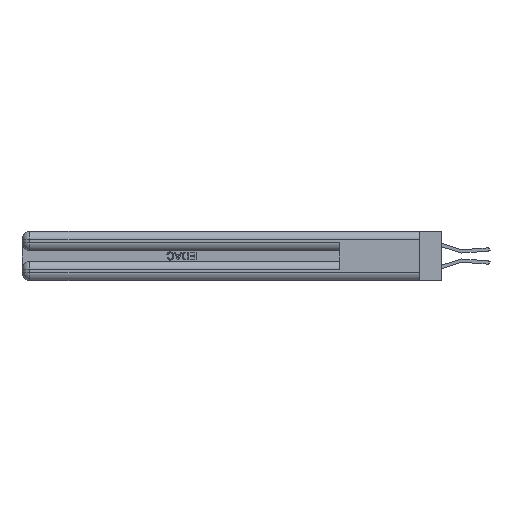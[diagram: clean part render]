
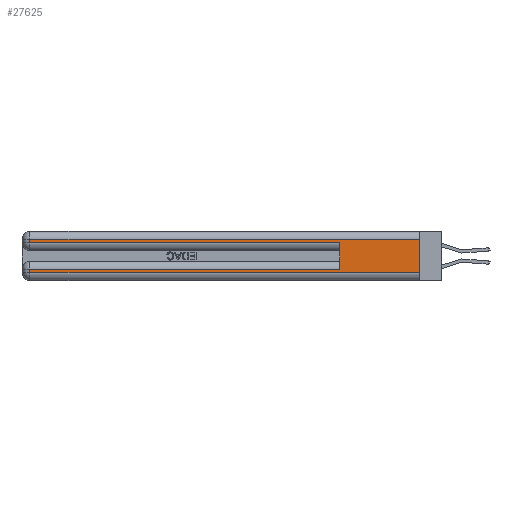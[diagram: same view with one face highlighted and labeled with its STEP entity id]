
A CAD part, left-side view. The second image highlights one B-rep face of the part: STEP entity #27625.
In plain terms, the highlighted planar face has unit normal (-1, 0, 0).
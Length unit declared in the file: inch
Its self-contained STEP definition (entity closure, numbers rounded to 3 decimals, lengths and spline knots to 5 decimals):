
#593 = VECTOR ( 'NONE', #5340, 39.37008 ) ;
#1022 = EDGE_CURVE ( 'NONE', #13051, #31233, #8066, .T. ) ;
#1693 = LINE ( 'NONE', #26097, #593 ) ;
#4827 = LINE ( 'NONE', #14614, #22151 ) ;
#4850 = CARTESIAN_POINT ( 'NONE',  ( 0., 0., 0.06 ) ) ;
#5340 = DIRECTION ( 'NONE',  ( 0., 0., -1. ) ) ;
#6098 = VECTOR ( 'NONE', #33694, 39.37008 ) ;
#6154 = ORIENTED_EDGE ( 'NONE', *, *, #6238, .T. ) ;
#6183 = VECTOR ( 'NONE', #44183, 39.37008 ) ;
#6238 = EDGE_CURVE ( 'NONE', #12537, #31115, #41715, .T. ) ;
#7185 = EDGE_CURVE ( 'NONE', #34861, #31233, #4827, .T. ) ;
#8066 = LINE ( 'NONE', #21139, #43744 ) ;
#8186 = ORIENTED_EDGE ( 'NONE', *, *, #37562, .F. ) ;
#10264 = CARTESIAN_POINT ( 'NONE',  ( 0., 0., 0.37 ) ) ;
#10406 = EDGE_LOOP ( 'NONE', ( #8186, #20085, #37996, #13645, #25565, #37518, #39146, #6154 ) ) ;
#10673 = VERTEX_POINT ( 'NONE', #22698 ) ;
#10731 = VERTEX_POINT ( 'NONE', #16223 ) ;
#11060 = CARTESIAN_POINT ( 'NONE',  ( 0., 2.94, 0.37 ) ) ;
#12537 = VERTEX_POINT ( 'NONE', #40251 ) ;
#13051 = VERTEX_POINT ( 'NONE', #29453 ) ;
#13645 = ORIENTED_EDGE ( 'NONE', *, *, #7185, .T. ) ;
#14118 = CARTESIAN_POINT ( 'NONE',  ( 0., 0., 0.085 ) ) ;
#14153 = VECTOR ( 'NONE', #23582, 39.37008 ) ;
#14243 = LINE ( 'NONE', #26737, #6098 ) ;
#14614 = CARTESIAN_POINT ( 'NONE',  ( 0., 0., 0.285 ) ) ;
#16223 = CARTESIAN_POINT ( 'NONE',  ( 0., 0., 0.31 ) ) ;
#16676 = CARTESIAN_POINT ( 'NONE',  ( 0., 2.94, 0.31 ) ) ;
#16988 = EDGE_CURVE ( 'NONE', #10673, #12537, #40811, .T. ) ;
#20000 = CARTESIAN_POINT ( 'NONE',  ( 0., 2.94, 0.37 ) ) ;
#20085 = ORIENTED_EDGE ( 'NONE', *, *, #32410, .T. ) ;
#20654 = DIRECTION ( 'NONE',  ( 1., 0., 0. ) ) ;
#21139 = CARTESIAN_POINT ( 'NONE',  ( 0., 0.6, 0.145 ) ) ;
#22151 = VECTOR ( 'NONE', #28343, 39.37008 ) ;
#22698 = CARTESIAN_POINT ( 'NONE',  ( 0., 2.94, 0.085 ) ) ;
#23582 = DIRECTION ( 'NONE',  ( 0., -1., 0. ) ) ;
#24001 = EDGE_CURVE ( 'NONE', #41924, #34861, #28791, .T. ) ;
#24778 = DIRECTION ( 'NONE',  ( 0., 0., 1. ) ) ;
#25565 = ORIENTED_EDGE ( 'NONE', *, *, #1022, .F. ) ;
#26097 = CARTESIAN_POINT ( 'NONE',  ( 0., 0., 0.37 ) ) ;
#26737 = CARTESIAN_POINT ( 'NONE',  ( 0., 0., 0.31 ) ) ;
#27625 = ADVANCED_FACE ( 'NONE', ( #40016 ), #41372, .F. ) ;
#27998 = DIRECTION ( 'NONE',  ( 0., 1., 0. ) ) ;
#28256 = DIRECTION ( 'NONE',  ( 0., 0., -1. ) ) ;
#28343 = DIRECTION ( 'NONE',  ( 0., -1., 0. ) ) ;
#28399 = CARTESIAN_POINT ( 'NONE',  ( 0., 2.94, 0.285 ) ) ;
#28791 = LINE ( 'NONE', #11060, #36939 ) ;
#29159 = EDGE_CURVE ( 'NONE', #13051, #10673, #42594, .T. ) ;
#29453 = CARTESIAN_POINT ( 'NONE',  ( 0., 0.6, 0.085 ) ) ;
#31115 = VERTEX_POINT ( 'NONE', #4850 ) ;
#31233 = VERTEX_POINT ( 'NONE', #36505 ) ;
#32410 = EDGE_CURVE ( 'NONE', #10731, #41924, #14243, .T. ) ;
#33409 = VECTOR ( 'NONE', #27998, 39.37008 ) ;
#33694 = DIRECTION ( 'NONE',  ( 0., 1., 0. ) ) ;
#34861 = VERTEX_POINT ( 'NONE', #28399 ) ;
#36505 = CARTESIAN_POINT ( 'NONE',  ( 0., 0.6, 0.285 ) ) ;
#36939 = VECTOR ( 'NONE', #28256, 39.37008 ) ;
#37518 = ORIENTED_EDGE ( 'NONE', *, *, #29159, .T. ) ;
#37562 = EDGE_CURVE ( 'NONE', #10731, #31115, #1693, .T. ) ;
#37996 = ORIENTED_EDGE ( 'NONE', *, *, #24001, .T. ) ;
#39146 = ORIENTED_EDGE ( 'NONE', *, *, #16988, .T. ) ;
#40016 = FACE_OUTER_BOUND ( 'NONE', #10406, .T. ) ;
#40251 = CARTESIAN_POINT ( 'NONE',  ( 0., 2.94, 0.06 ) ) ;
#40811 = LINE ( 'NONE', #20000, #6183 ) ;
#41372 = PLANE ( 'NONE',  #42147 ) ;
#41715 = LINE ( 'NONE', #44312, #14153 ) ;
#41924 = VERTEX_POINT ( 'NONE', #16676 ) ;
#42147 = AXIS2_PLACEMENT_3D ( 'NONE', #10264, #20654, #44862 ) ;
#42594 = LINE ( 'NONE', #14118, #33409 ) ;
#43744 = VECTOR ( 'NONE', #24778, 39.37008 ) ;
#44183 = DIRECTION ( 'NONE',  ( 0., 0., -1. ) ) ;
#44312 = CARTESIAN_POINT ( 'NONE',  ( 0., 0., 0.06 ) ) ;
#44862 = DIRECTION ( 'NONE',  ( 0., 0., -1. ) ) ;
